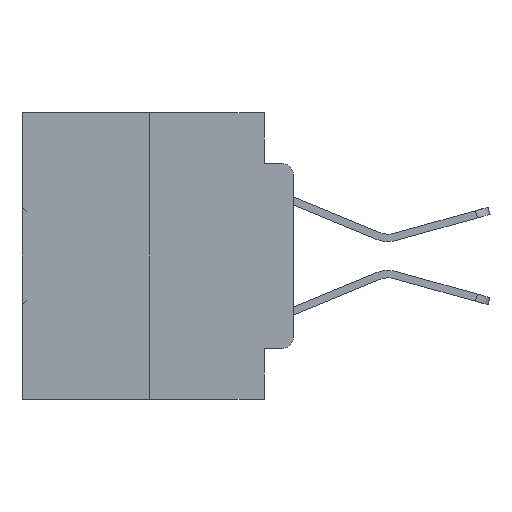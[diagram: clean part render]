
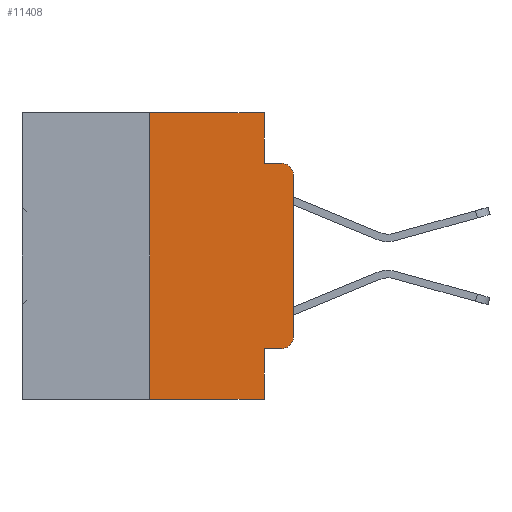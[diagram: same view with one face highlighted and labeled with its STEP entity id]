
A CAD part, left-side view. The second image highlights one B-rep face of the part: STEP entity #11408.
In plain terms, the highlighted planar face has unit normal (-1, 0, 0).
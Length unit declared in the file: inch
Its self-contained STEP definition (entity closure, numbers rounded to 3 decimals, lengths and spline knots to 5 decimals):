
#54 = VERTEX_POINT ( 'NONE', #29240 ) ;
#173 = EDGE_LOOP ( 'NONE', ( #11283, #12002, #15429, #20079, #22098, #6966, #829, #15756, #6414, #13053 ) ) ;
#422 = CARTESIAN_POINT ( 'NONE',  ( 0., 0.25, 0. ) ) ;
#753 = VERTEX_POINT ( 'NONE', #3817 ) ;
#829 = ORIENTED_EDGE ( 'NONE', *, *, #26625, .T. ) ;
#910 = LINE ( 'NONE', #9410, #9060 ) ;
#1033 = AXIS2_PLACEMENT_3D ( 'NONE', #34100, #18368, #1970 ) ;
#1294 = VERTEX_POINT ( 'NONE', #1761 ) ;
#1761 = CARTESIAN_POINT ( 'NONE',  ( 0., 0.02, -0.0885 ) ) ;
#1882 = LINE ( 'NONE', #12503, #29781 ) ;
#1970 = DIRECTION ( 'NONE',  ( 0., 0., -1. ) ) ;
#2149 = AXIS2_PLACEMENT_3D ( 'NONE', #2321, #21408, #5083 ) ;
#2321 = CARTESIAN_POINT ( 'NONE',  ( 0., 0.02, -0.3915 ) ) ;
#2979 = VERTEX_POINT ( 'NONE', #25205 ) ;
#3339 = CARTESIAN_POINT ( 'NONE',  ( 0., 0.051, 0. ) ) ;
#3587 = EDGE_CURVE ( 'NONE', #2979, #753, #18878, .T. ) ;
#3817 = CARTESIAN_POINT ( 'NONE',  ( 0., 0.02, -0.4115 ) ) ;
#4681 = CARTESIAN_POINT ( 'NONE',  ( 0., 0., 0. ) ) ;
#5083 = DIRECTION ( 'NONE',  ( 0., 0., -1. ) ) ;
#5428 = VERTEX_POINT ( 'NONE', #27531 ) ;
#5557 = VERTEX_POINT ( 'NONE', #34749 ) ;
#5650 = CIRCLE ( 'NONE', #1033, 0.02 ) ;
#5771 = LINE ( 'NONE', #12372, #19416 ) ;
#6178 = VECTOR ( 'NONE', #30901, 39.37008 ) ;
#6414 = ORIENTED_EDGE ( 'NONE', *, *, #3587, .T. ) ;
#6556 = CARTESIAN_POINT ( 'NONE',  ( 0., 0.473, 0. ) ) ;
#6966 = ORIENTED_EDGE ( 'NONE', *, *, #31978, .F. ) ;
#7942 = EDGE_CURVE ( 'NONE', #26768, #30737, #1882, .T. ) ;
#8734 = CARTESIAN_POINT ( 'NONE',  ( 0., 0.473, 0. ) ) ;
#9060 = VECTOR ( 'NONE', #25743, 39.37008 ) ;
#9410 = CARTESIAN_POINT ( 'NONE',  ( 0., 0.473, -0.5 ) ) ;
#10208 = DIRECTION ( 'NONE',  ( 0., 0., 1. ) ) ;
#11283 = ORIENTED_EDGE ( 'NONE', *, *, #16643, .T. ) ;
#11408 = ADVANCED_FACE ( 'NONE', ( #26673 ), #14248, .F. ) ;
#11625 = EDGE_CURVE ( 'NONE', #30737, #1294, #27747, .T. ) ;
#11767 = LINE ( 'NONE', #32982, #12625 ) ;
#12002 = ORIENTED_EDGE ( 'NONE', *, *, #20520, .T. ) ;
#12372 = CARTESIAN_POINT ( 'NONE',  ( 0., 0.25, 0. ) ) ;
#12503 = CARTESIAN_POINT ( 'NONE',  ( 0., 0.051, 0. ) ) ;
#12504 = VECTOR ( 'NONE', #15927, 39.37008 ) ;
#12625 = VECTOR ( 'NONE', #17162, 39.37008 ) ;
#13053 = ORIENTED_EDGE ( 'NONE', *, *, #29608, .T. ) ;
#13953 = VECTOR ( 'NONE', #10208, 39.37008 ) ;
#14248 = PLANE ( 'NONE',  #25670 ) ;
#14614 = DIRECTION ( 'NONE',  ( 0., -1., 0. ) ) ;
#14959 = CARTESIAN_POINT ( 'NONE',  ( 0., 0.051, -0.0885 ) ) ;
#15149 = DIRECTION ( 'NONE',  ( 0., 0., 1. ) ) ;
#15272 = DIRECTION ( 'NONE',  ( 0., 0., -1. ) ) ;
#15365 = CARTESIAN_POINT ( 'NONE',  ( 0., 0.25, -0.5 ) ) ;
#15429 = ORIENTED_EDGE ( 'NONE', *, *, #11625, .F. ) ;
#15756 = ORIENTED_EDGE ( 'NONE', *, *, #18924, .F. ) ;
#15927 = DIRECTION ( 'NONE',  ( 0., -1., 0. ) ) ;
#16111 = CARTESIAN_POINT ( 'NONE',  ( 0., 0.051, -0.4115 ) ) ;
#16643 = EDGE_CURVE ( 'NONE', #5428, #5557, #21161, .T. ) ;
#16991 = DIRECTION ( 'NONE',  ( 0., 0., -1. ) ) ;
#17162 = DIRECTION ( 'NONE',  ( 0., 0., -1. ) ) ;
#18368 = DIRECTION ( 'NONE',  ( -1., 0., 0. ) ) ;
#18878 = LINE ( 'NONE', #16111, #12504 ) ;
#18924 = EDGE_CURVE ( 'NONE', #2979, #54, #11767, .T. ) ;
#19416 = VECTOR ( 'NONE', #15149, 39.37008 ) ;
#20079 = ORIENTED_EDGE ( 'NONE', *, *, #7942, .F. ) ;
#20520 = EDGE_CURVE ( 'NONE', #5557, #1294, #5650, .T. ) ;
#21161 = LINE ( 'NONE', #4681, #13953 ) ;
#21408 = DIRECTION ( 'NONE',  ( -1., 0., 0. ) ) ;
#22076 = VECTOR ( 'NONE', #14614, 39.37008 ) ;
#22098 = ORIENTED_EDGE ( 'NONE', *, *, #22954, .F. ) ;
#22419 = VERTEX_POINT ( 'NONE', #15365 ) ;
#22936 = LINE ( 'NONE', #6556, #22076 ) ;
#22954 = EDGE_CURVE ( 'NONE', #24554, #26768, #22936, .T. ) ;
#24554 = VERTEX_POINT ( 'NONE', #422 ) ;
#25205 = CARTESIAN_POINT ( 'NONE',  ( 0., 0.051, -0.4115 ) ) ;
#25670 = AXIS2_PLACEMENT_3D ( 'NONE', #8734, #32808, #16991 ) ;
#25743 = DIRECTION ( 'NONE',  ( 0., -1., 0. ) ) ;
#26027 = CARTESIAN_POINT ( 'NONE',  ( 0., 0.051, -0.0885 ) ) ;
#26625 = EDGE_CURVE ( 'NONE', #22419, #54, #910, .T. ) ;
#26673 = FACE_OUTER_BOUND ( 'NONE', #173, .T. ) ;
#26768 = VERTEX_POINT ( 'NONE', #3339 ) ;
#27531 = CARTESIAN_POINT ( 'NONE',  ( 0., 0., -0.3915 ) ) ;
#27747 = LINE ( 'NONE', #14959, #6178 ) ;
#29240 = CARTESIAN_POINT ( 'NONE',  ( 0., 0.051, -0.5 ) ) ;
#29608 = EDGE_CURVE ( 'NONE', #753, #5428, #31558, .T. ) ;
#29781 = VECTOR ( 'NONE', #15272, 39.37008 ) ;
#30737 = VERTEX_POINT ( 'NONE', #26027 ) ;
#30901 = DIRECTION ( 'NONE',  ( 0., -1., 0. ) ) ;
#31558 = CIRCLE ( 'NONE', #2149, 0.02 ) ;
#31978 = EDGE_CURVE ( 'NONE', #22419, #24554, #5771, .T. ) ;
#32808 = DIRECTION ( 'NONE',  ( 1., 0., 0. ) ) ;
#32982 = CARTESIAN_POINT ( 'NONE',  ( 0., 0.051, 0. ) ) ;
#34100 = CARTESIAN_POINT ( 'NONE',  ( 0., 0.02, -0.1085 ) ) ;
#34749 = CARTESIAN_POINT ( 'NONE',  ( 0., 0., -0.1085 ) ) ;
